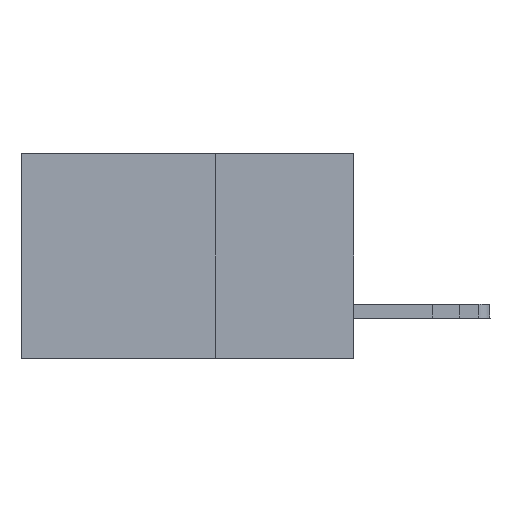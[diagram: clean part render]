
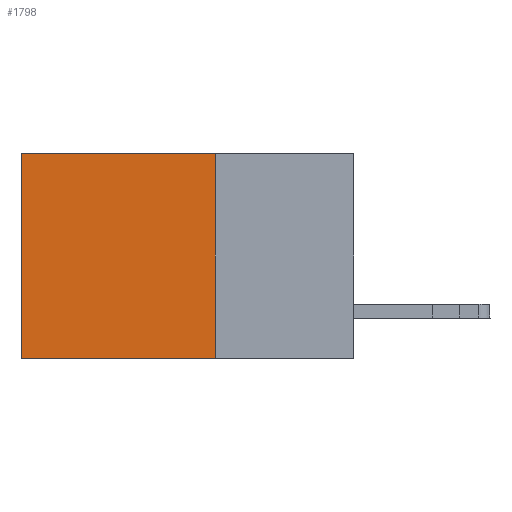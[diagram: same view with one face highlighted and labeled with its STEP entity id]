
A CAD part, left-side view. The second image highlights one B-rep face of the part: STEP entity #1798.
In plain terms, the highlighted planar face has unit normal (-1, 0, 0).
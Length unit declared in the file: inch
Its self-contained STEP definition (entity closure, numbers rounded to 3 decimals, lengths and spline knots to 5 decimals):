
#439 = DIRECTION ( 'NONE',  ( 0., 1., 0. ) ) ;
#1798 = ADVANCED_FACE ( 'NONE', ( #11939 ), #12434, .F. ) ;
#2680 = AXIS2_PLACEMENT_3D ( 'NONE', #18754, #20910, #10152 ) ;
#3856 = DIRECTION ( 'NONE',  ( 0., 0., -1. ) ) ;
#4634 = VECTOR ( 'NONE', #15203, 39.37008 ) ;
#4780 = LINE ( 'NONE', #11081, #26593 ) ;
#4923 = EDGE_CURVE ( 'NONE', #22594, #26544, #22752, .T. ) ;
#5378 = CARTESIAN_POINT ( 'NONE',  ( 0.2875, 0.6, 0. ) ) ;
#5728 = CARTESIAN_POINT ( 'NONE',  ( 0.2875, 0.25, 0. ) ) ;
#5890 = VECTOR ( 'NONE', #23913, 39.37008 ) ;
#5904 = EDGE_LOOP ( 'NONE', ( #8767, #6892, #9402, #25135 ) ) ;
#6892 = ORIENTED_EDGE ( 'NONE', *, *, #4923, .F. ) ;
#8761 = VERTEX_POINT ( 'NONE', #5728 ) ;
#8767 = ORIENTED_EDGE ( 'NONE', *, *, #13452, .T. ) ;
#9402 = ORIENTED_EDGE ( 'NONE', *, *, #23408, .F. ) ;
#9850 = EDGE_CURVE ( 'NONE', #8761, #26410, #4780, .T. ) ;
#10152 = DIRECTION ( 'NONE',  ( 0., 0., -1. ) ) ;
#10367 = LINE ( 'NONE', #16511, #25431 ) ;
#11018 = CARTESIAN_POINT ( 'NONE',  ( 0.2875, 0.6, 0. ) ) ;
#11081 = CARTESIAN_POINT ( 'NONE',  ( 0.2875, 0.25, 0. ) ) ;
#11939 = FACE_OUTER_BOUND ( 'NONE', #5904, .T. ) ;
#12434 = PLANE ( 'NONE',  #2680 ) ;
#13452 = EDGE_CURVE ( 'NONE', #26410, #26544, #17962, .T. ) ;
#15203 = DIRECTION ( 'NONE',  ( 0., 1., 0. ) ) ;
#15694 = CARTESIAN_POINT ( 'NONE',  ( 0.2875, 0.25, -0.37 ) ) ;
#16511 = CARTESIAN_POINT ( 'NONE',  ( 0.2875, 0.25, 0. ) ) ;
#17278 = CARTESIAN_POINT ( 'NONE',  ( 0.2875, 0.6, -0.37 ) ) ;
#17962 = LINE ( 'NONE', #11018, #5890 ) ;
#18754 = CARTESIAN_POINT ( 'NONE',  ( 0.2875, 0.25, 0. ) ) ;
#20910 = DIRECTION ( 'NONE',  ( 1., 0., 0. ) ) ;
#22594 = VERTEX_POINT ( 'NONE', #24305 ) ;
#22752 = LINE ( 'NONE', #15694, #4634 ) ;
#23408 = EDGE_CURVE ( 'NONE', #8761, #22594, #10367, .T. ) ;
#23913 = DIRECTION ( 'NONE',  ( 0., 0., -1. ) ) ;
#24305 = CARTESIAN_POINT ( 'NONE',  ( 0.2875, 0.25, -0.37 ) ) ;
#25135 = ORIENTED_EDGE ( 'NONE', *, *, #9850, .T. ) ;
#25431 = VECTOR ( 'NONE', #3856, 39.37008 ) ;
#26410 = VERTEX_POINT ( 'NONE', #5378 ) ;
#26544 = VERTEX_POINT ( 'NONE', #17278 ) ;
#26593 = VECTOR ( 'NONE', #439, 39.37008 ) ;
